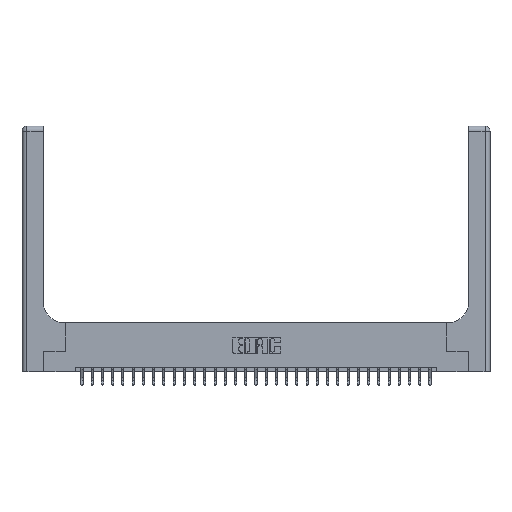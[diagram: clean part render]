
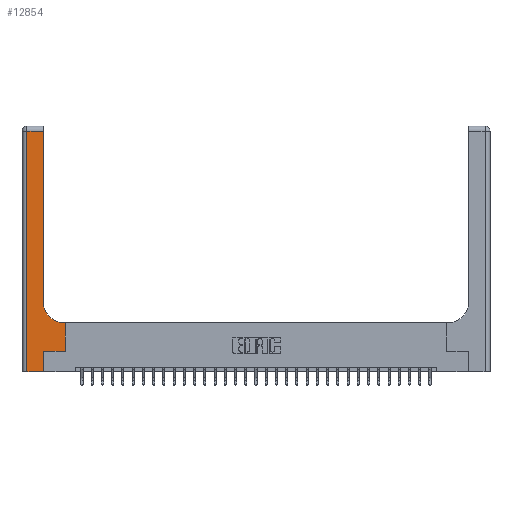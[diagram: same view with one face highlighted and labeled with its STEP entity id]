
A CAD part, top view. The second image highlights one B-rep face of the part: STEP entity #12854.
In plain terms, the highlighted planar face has unit normal (0, 0, 1).
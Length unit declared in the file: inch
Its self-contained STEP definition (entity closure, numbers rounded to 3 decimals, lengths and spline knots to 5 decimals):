
#311 = CARTESIAN_POINT ( 'NONE',  ( 0.06, 2.94, 0.37 ) ) ;
#375 = EDGE_CURVE ( 'NONE', #23263, #9249, #17331, .T. ) ;
#1006 = DIRECTION ( 'NONE',  ( 0., 1., 0. ) ) ;
#1551 = CARTESIAN_POINT ( 'NONE',  ( 0., 2.94, 0.37 ) ) ;
#1779 = CARTESIAN_POINT ( 'NONE',  ( 0.265, 0., 0.37 ) ) ;
#1789 = DIRECTION ( 'NONE',  ( 0., 0., -1. ) ) ;
#2134 = ORIENTED_EDGE ( 'NONE', *, *, #5062, .T. ) ;
#2214 = CARTESIAN_POINT ( 'NONE',  ( 0., 3., 0.37 ) ) ;
#2232 = CARTESIAN_POINT ( 'NONE',  ( 0.265, 0., 0.37 ) ) ;
#2260 = CIRCLE ( 'NONE', #16168, 0.25 ) ;
#2731 = DIRECTION ( 'NONE',  ( -1., 0., 0. ) ) ;
#2766 = EDGE_CURVE ( 'NONE', #4716, #4133, #13649, .T. ) ;
#3153 = ORIENTED_EDGE ( 'NONE', *, *, #15234, .T. ) ;
#3557 = CARTESIAN_POINT ( 'NONE',  ( 0., 0., 0.37 ) ) ;
#3656 = CARTESIAN_POINT ( 'NONE',  ( 0.06, 3., 0.37 ) ) ;
#4056 = VECTOR ( 'NONE', #26628, 39.37008 ) ;
#4133 = VERTEX_POINT ( 'NONE', #21534 ) ;
#4487 = VECTOR ( 'NONE', #11761, 39.37008 ) ;
#4716 = VERTEX_POINT ( 'NONE', #1779 ) ;
#5062 = EDGE_CURVE ( 'NONE', #12892, #17141, #7613, .T. ) ;
#5415 = VECTOR ( 'NONE', #15610, 39.37008 ) ;
#6608 = AXIS2_PLACEMENT_3D ( 'NONE', #2214, #6731, #18136 ) ;
#6678 = LINE ( 'NONE', #20342, #4487 ) ;
#6731 = DIRECTION ( 'NONE',  ( 0., 0., -1. ) ) ;
#6927 = EDGE_LOOP ( 'NONE', ( #2134, #20161, #23088, #27447, #22613, #9337, #26660, #3153, #27945 ) ) ;
#7613 = LINE ( 'NONE', #14527, #23165 ) ;
#8137 = EDGE_CURVE ( 'NONE', #4133, #9867, #6678, .T. ) ;
#8964 = FACE_OUTER_BOUND ( 'NONE', #6927, .T. ) ;
#9249 = VERTEX_POINT ( 'NONE', #26797 ) ;
#9337 = ORIENTED_EDGE ( 'NONE', *, *, #8137, .T. ) ;
#9431 = VECTOR ( 'NONE', #12577, 39.37008 ) ;
#9867 = VERTEX_POINT ( 'NONE', #27797 ) ;
#10930 = VECTOR ( 'NONE', #2731, 39.37008 ) ;
#11085 = PLANE ( 'NONE',  #6608 ) ;
#11743 = CARTESIAN_POINT ( 'NONE',  ( 0.528, 0.6, 0.37 ) ) ;
#11761 = DIRECTION ( 'NONE',  ( 1., 0., 0. ) ) ;
#12577 = DIRECTION ( 'NONE',  ( 1., 0., 0. ) ) ;
#12854 = ADVANCED_FACE ( 'NONE', ( #8964 ), #11085, .F. ) ;
#12892 = VERTEX_POINT ( 'NONE', #17988 ) ;
#13640 = EDGE_CURVE ( 'NONE', #17141, #23263, #24672, .T. ) ;
#13649 = LINE ( 'NONE', #2232, #5415 ) ;
#13822 = VERTEX_POINT ( 'NONE', #11743 ) ;
#14527 = CARTESIAN_POINT ( 'NONE',  ( 0.26, 3., 0.37 ) ) ;
#14552 = CARTESIAN_POINT ( 'NONE',  ( 0.26, 2.94, 0.37 ) ) ;
#15234 = EDGE_CURVE ( 'NONE', #13822, #20599, #16408, .T. ) ;
#15610 = DIRECTION ( 'NONE',  ( 0., 1., 0. ) ) ;
#15611 = DIRECTION ( 'NONE',  ( 1., 0., 0. ) ) ;
#16168 = AXIS2_PLACEMENT_3D ( 'NONE', #18158, #1789, #15611 ) ;
#16408 = LINE ( 'NONE', #25547, #10930 ) ;
#17141 = VERTEX_POINT ( 'NONE', #14552 ) ;
#17331 = LINE ( 'NONE', #3656, #4056 ) ;
#17371 = LINE ( 'NONE', #3557, #9431 ) ;
#17988 = CARTESIAN_POINT ( 'NONE',  ( 0.26, 0.85, 0.37 ) ) ;
#18105 = VECTOR ( 'NONE', #26495, 39.37008 ) ;
#18136 = DIRECTION ( 'NONE',  ( -1., 0., 0. ) ) ;
#18158 = CARTESIAN_POINT ( 'NONE',  ( 0.51, 0.85, 0.37 ) ) ;
#19443 = LINE ( 'NONE', #28585, #18105 ) ;
#19869 = DIRECTION ( 'NONE',  ( -1., 0., 0. ) ) ;
#20161 = ORIENTED_EDGE ( 'NONE', *, *, #13640, .T. ) ;
#20342 = CARTESIAN_POINT ( 'NONE',  ( 0.265, 0.25, 0.37 ) ) ;
#20581 = CARTESIAN_POINT ( 'NONE',  ( 0.51, 0.6, 0.37 ) ) ;
#20599 = VERTEX_POINT ( 'NONE', #20581 ) ;
#21534 = CARTESIAN_POINT ( 'NONE',  ( 0.265, 0.25, 0.37 ) ) ;
#22613 = ORIENTED_EDGE ( 'NONE', *, *, #2766, .T. ) ;
#23088 = ORIENTED_EDGE ( 'NONE', *, *, #375, .T. ) ;
#23165 = VECTOR ( 'NONE', #1006, 39.37008 ) ;
#23263 = VERTEX_POINT ( 'NONE', #311 ) ;
#24373 = EDGE_CURVE ( 'NONE', #20599, #12892, #2260, .T. ) ;
#24539 = EDGE_CURVE ( 'NONE', #9249, #4716, #17371, .T. ) ;
#24672 = LINE ( 'NONE', #1551, #27641 ) ;
#25031 = EDGE_CURVE ( 'NONE', #9867, #13822, #19443, .T. ) ;
#25547 = CARTESIAN_POINT ( 'NONE',  ( 0.26, 0.6, 0.37 ) ) ;
#26495 = DIRECTION ( 'NONE',  ( 0., 1., 0. ) ) ;
#26628 = DIRECTION ( 'NONE',  ( 0., -1., 0. ) ) ;
#26660 = ORIENTED_EDGE ( 'NONE', *, *, #25031, .T. ) ;
#26797 = CARTESIAN_POINT ( 'NONE',  ( 0.06, 0., 0.37 ) ) ;
#27447 = ORIENTED_EDGE ( 'NONE', *, *, #24539, .T. ) ;
#27641 = VECTOR ( 'NONE', #19869, 39.37008 ) ;
#27797 = CARTESIAN_POINT ( 'NONE',  ( 0.528, 0.25, 0.37 ) ) ;
#27945 = ORIENTED_EDGE ( 'NONE', *, *, #24373, .T. ) ;
#28585 = CARTESIAN_POINT ( 'NONE',  ( 0.528, 0.25, 0.37 ) ) ;
